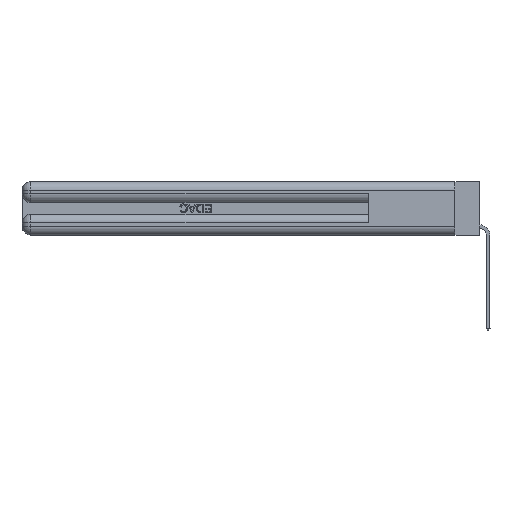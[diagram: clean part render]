
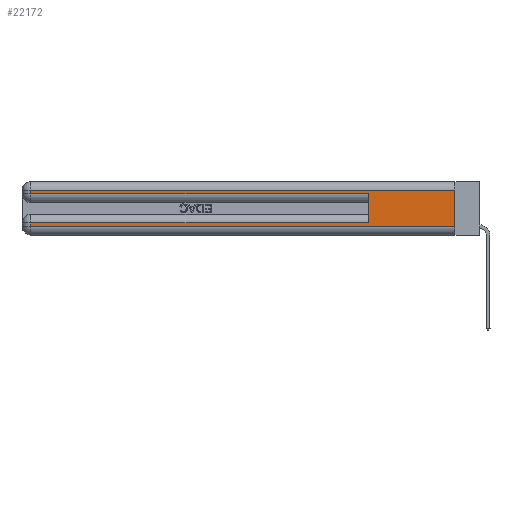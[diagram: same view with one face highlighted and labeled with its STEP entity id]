
A CAD part, left-side view. The second image highlights one B-rep face of the part: STEP entity #22172.
In plain terms, the highlighted planar face has unit normal (-1, 0, 0).
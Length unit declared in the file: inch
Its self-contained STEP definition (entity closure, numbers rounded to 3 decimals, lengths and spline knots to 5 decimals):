
#413 = ORIENTED_EDGE ( 'NONE', *, *, #537, .F. ) ;
#537 = EDGE_CURVE ( 'NONE', #24179, #19845, #19879, .T. ) ;
#594 = EDGE_CURVE ( 'NONE', #4277, #19845, #6539, .T. ) ;
#898 = DIRECTION ( 'NONE',  ( 0., -1., 0. ) ) ;
#2200 = DIRECTION ( 'NONE',  ( 0., 0., -1. ) ) ;
#2503 = LINE ( 'NONE', #18311, #19649 ) ;
#2539 = LINE ( 'NONE', #12482, #24973 ) ;
#2862 = EDGE_CURVE ( 'NONE', #15907, #6341, #14545, .T. ) ;
#3033 = CARTESIAN_POINT ( 'NONE',  ( 0., 0., 0.31 ) ) ;
#3606 = AXIS2_PLACEMENT_3D ( 'NONE', #29026, #15637, #2200 ) ;
#3789 = CARTESIAN_POINT ( 'NONE',  ( 0., 2.94, 0.285 ) ) ;
#3837 = LINE ( 'NONE', #19838, #9029 ) ;
#4277 = VERTEX_POINT ( 'NONE', #3789 ) ;
#4894 = DIRECTION ( 'NONE',  ( 0., 0., -1. ) ) ;
#5314 = CARTESIAN_POINT ( 'NONE',  ( 0., 0., 0.06 ) ) ;
#5658 = VERTEX_POINT ( 'NONE', #8562 ) ;
#5715 = EDGE_CURVE ( 'NONE', #15907, #5658, #10443, .T. ) ;
#6341 = VERTEX_POINT ( 'NONE', #21372 ) ;
#6539 = LINE ( 'NONE', #17829, #18495 ) ;
#7568 = VECTOR ( 'NONE', #898, 39.37008 ) ;
#7745 = ORIENTED_EDGE ( 'NONE', *, *, #2862, .F. ) ;
#8562 = CARTESIAN_POINT ( 'NONE',  ( 0., 2.94, 0.31 ) ) ;
#8652 = DIRECTION ( 'NONE',  ( 0., 1., 0. ) ) ;
#9029 = VECTOR ( 'NONE', #8652, 39.37008 ) ;
#9135 = CARTESIAN_POINT ( 'NONE',  ( 0., 0., 0.31 ) ) ;
#9145 = ORIENTED_EDGE ( 'NONE', *, *, #12644, .T. ) ;
#9324 = DIRECTION ( 'NONE',  ( 0., 1., 0. ) ) ;
#9406 = CARTESIAN_POINT ( 'NONE',  ( 0., 2.94, 0.06 ) ) ;
#10443 = LINE ( 'NONE', #9135, #27663 ) ;
#11121 = CARTESIAN_POINT ( 'NONE',  ( 0., 0.6, 0.085 ) ) ;
#11535 = EDGE_CURVE ( 'NONE', #19122, #23149, #2539, .T. ) ;
#11897 = EDGE_LOOP ( 'NONE', ( #7745, #13742, #24968, #18294, #413, #9145, #18358, #12365 ) ) ;
#12365 = ORIENTED_EDGE ( 'NONE', *, *, #13652, .T. ) ;
#12482 = CARTESIAN_POINT ( 'NONE',  ( 0., 2.94, 0.37 ) ) ;
#12644 = EDGE_CURVE ( 'NONE', #24179, #19122, #3837, .T. ) ;
#13011 = DIRECTION ( 'NONE',  ( 0., 0., 1. ) ) ;
#13652 = EDGE_CURVE ( 'NONE', #23149, #6341, #14994, .T. ) ;
#13742 = ORIENTED_EDGE ( 'NONE', *, *, #5715, .T. ) ;
#14545 = LINE ( 'NONE', #26065, #19776 ) ;
#14994 = LINE ( 'NONE', #5314, #7568 ) ;
#15637 = DIRECTION ( 'NONE',  ( 1., 0., 0. ) ) ;
#15907 = VERTEX_POINT ( 'NONE', #3033 ) ;
#16035 = CARTESIAN_POINT ( 'NONE',  ( 0., 0.6, 0.285 ) ) ;
#17015 = FACE_OUTER_BOUND ( 'NONE', #11897, .T. ) ;
#17541 = CARTESIAN_POINT ( 'NONE',  ( 0., 2.94, 0.085 ) ) ;
#17829 = CARTESIAN_POINT ( 'NONE',  ( 0., 0., 0.285 ) ) ;
#18294 = ORIENTED_EDGE ( 'NONE', *, *, #594, .T. ) ;
#18311 = CARTESIAN_POINT ( 'NONE',  ( 0., 2.94, 0.37 ) ) ;
#18358 = ORIENTED_EDGE ( 'NONE', *, *, #11535, .T. ) ;
#18495 = VECTOR ( 'NONE', #22327, 39.37008 ) ;
#19122 = VERTEX_POINT ( 'NONE', #17541 ) ;
#19185 = VECTOR ( 'NONE', #13011, 39.37008 ) ;
#19649 = VECTOR ( 'NONE', #4894, 39.37008 ) ;
#19776 = VECTOR ( 'NONE', #23988, 39.37008 ) ;
#19838 = CARTESIAN_POINT ( 'NONE',  ( 0., 0., 0.085 ) ) ;
#19845 = VERTEX_POINT ( 'NONE', #16035 ) ;
#19879 = LINE ( 'NONE', #26570, #19185 ) ;
#21372 = CARTESIAN_POINT ( 'NONE',  ( 0., 0., 0.06 ) ) ;
#22172 = ADVANCED_FACE ( 'NONE', ( #17015 ), #24524, .F. ) ;
#22327 = DIRECTION ( 'NONE',  ( 0., -1., 0. ) ) ;
#23149 = VERTEX_POINT ( 'NONE', #9406 ) ;
#23988 = DIRECTION ( 'NONE',  ( 0., 0., -1. ) ) ;
#24179 = VERTEX_POINT ( 'NONE', #11121 ) ;
#24299 = EDGE_CURVE ( 'NONE', #5658, #4277, #2503, .T. ) ;
#24524 = PLANE ( 'NONE',  #3606 ) ;
#24968 = ORIENTED_EDGE ( 'NONE', *, *, #24299, .T. ) ;
#24973 = VECTOR ( 'NONE', #25940, 39.37008 ) ;
#25940 = DIRECTION ( 'NONE',  ( 0., 0., -1. ) ) ;
#26065 = CARTESIAN_POINT ( 'NONE',  ( 0., 0., 0.37 ) ) ;
#26570 = CARTESIAN_POINT ( 'NONE',  ( 0., 0.6, 0.145 ) ) ;
#27663 = VECTOR ( 'NONE', #9324, 39.37008 ) ;
#29026 = CARTESIAN_POINT ( 'NONE',  ( 0., 0., 0.37 ) ) ;
